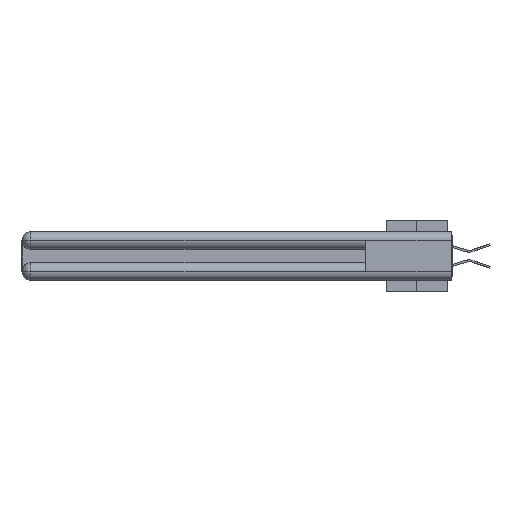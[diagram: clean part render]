
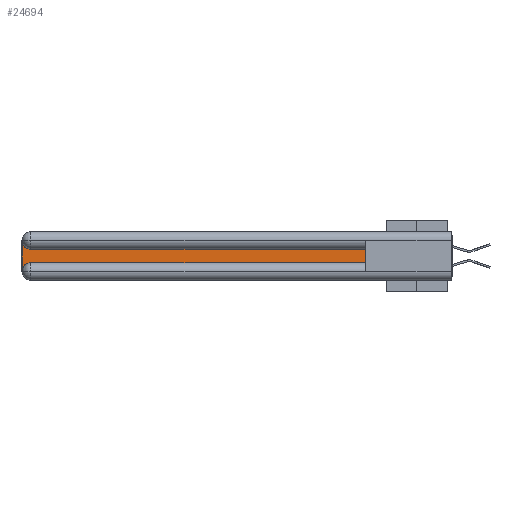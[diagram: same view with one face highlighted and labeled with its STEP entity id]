
A CAD part, left-side view. The second image highlights one B-rep face of the part: STEP entity #24694.
In plain terms, the highlighted planar face has unit normal (-1, 0, 0).
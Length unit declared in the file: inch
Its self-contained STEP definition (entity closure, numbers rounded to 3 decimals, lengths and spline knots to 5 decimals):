
#505 = VERTEX_POINT ( 'NONE', #16518 ) ;
#1304 = EDGE_CURVE ( 'NONE', #22653, #30185, #2659, .T. ) ;
#1414 = DIRECTION ( 'NONE',  ( 0., 0., 1. ) ) ;
#1431 = EDGE_CURVE ( 'NONE', #505, #14748, #35384, .T. ) ;
#1572 = CARTESIAN_POINT ( 'NONE',  ( 0.075, 3., -0.2775 ) ) ;
#2389 = ORIENTED_EDGE ( 'NONE', *, *, #11958, .T. ) ;
#2659 = CIRCLE ( 'NONE', #10527, 0.06 ) ;
#4374 = LINE ( 'NONE', #32403, #14312 ) ;
#5531 = VECTOR ( 'NONE', #33474, 39.37008 ) ;
#5854 = DIRECTION ( 'NONE',  ( 1., 0., 0. ) ) ;
#7335 = CARTESIAN_POINT ( 'NONE',  ( 0.075, 0.6, -0.1225 ) ) ;
#7854 = ORIENTED_EDGE ( 'NONE', *, *, #33456, .T. ) ;
#8651 = DIRECTION ( 'NONE',  ( 1., 0., 0. ) ) ;
#9196 = VERTEX_POINT ( 'NONE', #13449 ) ;
#9926 = VECTOR ( 'NONE', #33520, 39.37008 ) ;
#10527 = AXIS2_PLACEMENT_3D ( 'NONE', #44215, #8651, #25822 ) ;
#11958 = EDGE_CURVE ( 'NONE', #30185, #9196, #4374, .T. ) ;
#12058 = ORIENTED_EDGE ( 'NONE', *, *, #15870, .T. ) ;
#12625 = DIRECTION ( 'NONE',  ( 0., 0., -1. ) ) ;
#13319 = ORIENTED_EDGE ( 'NONE', *, *, #1431, .T. ) ;
#13449 = CARTESIAN_POINT ( 'NONE',  ( 0.075, 0.6, -0.2175 ) ) ;
#14312 = VECTOR ( 'NONE', #29459, 39.37008 ) ;
#14748 = VERTEX_POINT ( 'NONE', #34587 ) ;
#15870 = EDGE_CURVE ( 'NONE', #14748, #22653, #19390, .T. ) ;
#16518 = CARTESIAN_POINT ( 'NONE',  ( 0.075, 2.94, -0.1225 ) ) ;
#17616 = DIRECTION ( 'NONE',  ( 0., 0., -1. ) ) ;
#18452 = LINE ( 'NONE', #18973, #28938 ) ;
#18973 = CARTESIAN_POINT ( 'NONE',  ( 0.075, 0.6, -0.2175 ) ) ;
#19390 = LINE ( 'NONE', #26227, #9926 ) ;
#20132 = CARTESIAN_POINT ( 'NONE',  ( 0.075, 2.94, -0.0625 ) ) ;
#21191 = DIRECTION ( 'NONE',  ( 1., 0., 0. ) ) ;
#22653 = VERTEX_POINT ( 'NONE', #1572 ) ;
#23736 = FACE_OUTER_BOUND ( 'NONE', #44965, .T. ) ;
#24694 = ADVANCED_FACE ( 'NONE', ( #23736 ), #38826, .F. ) ;
#25822 = DIRECTION ( 'NONE',  ( 0., 0., -1. ) ) ;
#26227 = CARTESIAN_POINT ( 'NONE',  ( 0.075, 3., -0.2175 ) ) ;
#28938 = VECTOR ( 'NONE', #1414, 39.37008 ) ;
#28954 = VERTEX_POINT ( 'NONE', #7335 ) ;
#29459 = DIRECTION ( 'NONE',  ( 0., -1., 0. ) ) ;
#29831 = AXIS2_PLACEMENT_3D ( 'NONE', #20132, #5854, #12625 ) ;
#29924 = CARTESIAN_POINT ( 'NONE',  ( 0.075, 0.6, -0.1225 ) ) ;
#30185 = VERTEX_POINT ( 'NONE', #37048 ) ;
#30291 = EDGE_CURVE ( 'NONE', #28954, #505, #43175, .T. ) ;
#32403 = CARTESIAN_POINT ( 'NONE',  ( 0.075, 0.6, -0.2175 ) ) ;
#33456 = EDGE_CURVE ( 'NONE', #9196, #28954, #18452, .T. ) ;
#33474 = DIRECTION ( 'NONE',  ( 0., 1., 0. ) ) ;
#33520 = DIRECTION ( 'NONE',  ( 0., 0., -1. ) ) ;
#34587 = CARTESIAN_POINT ( 'NONE',  ( 0.075, 3., -0.0625 ) ) ;
#35384 = CIRCLE ( 'NONE', #29831, 0.06 ) ;
#37048 = CARTESIAN_POINT ( 'NONE',  ( 0.075, 2.94, -0.2175 ) ) ;
#37992 = ORIENTED_EDGE ( 'NONE', *, *, #1304, .T. ) ;
#38826 = PLANE ( 'NONE',  #40864 ) ;
#39149 = CARTESIAN_POINT ( 'NONE',  ( 0.075, 3., -0.1225 ) ) ;
#40864 = AXIS2_PLACEMENT_3D ( 'NONE', #39149, #21191, #17616 ) ;
#43175 = LINE ( 'NONE', #29924, #5531 ) ;
#44118 = ORIENTED_EDGE ( 'NONE', *, *, #30291, .T. ) ;
#44215 = CARTESIAN_POINT ( 'NONE',  ( 0.075, 2.94, -0.2775 ) ) ;
#44965 = EDGE_LOOP ( 'NONE', ( #44118, #13319, #12058, #37992, #2389, #7854 ) ) ;
